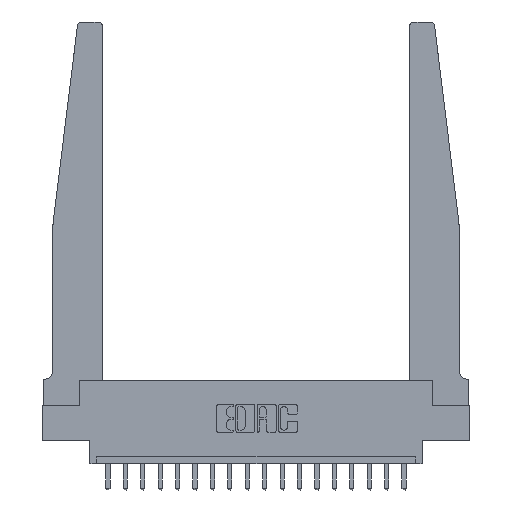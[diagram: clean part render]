
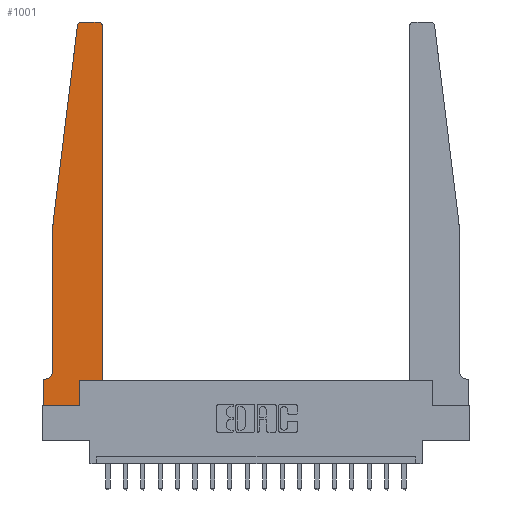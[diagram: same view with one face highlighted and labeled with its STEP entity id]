
A CAD part, top view. The second image highlights one B-rep face of the part: STEP entity #1001.
In plain terms, the highlighted planar face has unit normal (0, 0, 1).
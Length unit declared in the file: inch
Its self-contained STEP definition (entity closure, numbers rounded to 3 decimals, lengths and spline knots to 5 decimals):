
#189 = CARTESIAN_POINT ( 'NONE',  ( 0.425, 2.72, 0.37 ) ) ;
#307 = VERTEX_POINT ( 'NONE', #17129 ) ;
#1001 = ADVANCED_FACE ( 'NONE', ( #6312 ), #4808, .T. ) ;
#1049 = LINE ( 'NONE', #13398, #4897 ) ;
#1260 = EDGE_CURVE ( 'NONE', #4335, #16055, #1049, .T. ) ;
#1271 = ORIENTED_EDGE ( 'NONE', *, *, #1260, .T. ) ;
#1694 = ORIENTED_EDGE ( 'NONE', *, *, #8791, .T. ) ;
#1933 = LINE ( 'NONE', #2141, #8858 ) ;
#2081 = EDGE_CURVE ( 'NONE', #16055, #9278, #18483, .T. ) ;
#2141 = CARTESIAN_POINT ( 'NONE',  ( 0.065, 1.25, 0.37 ) ) ;
#2741 = CARTESIAN_POINT ( 'NONE',  ( 0.24675, 2.72367, 0.37 ) ) ;
#2771 = DIRECTION ( 'NONE',  ( 0., 1., 0. ) ) ;
#2878 = DIRECTION ( 'NONE',  ( 1., 0., 0. ) ) ;
#2990 = CARTESIAN_POINT ( 'NONE',  ( 0., 0., 0.37 ) ) ;
#3094 = DIRECTION ( 'NONE',  ( 0., -1., 0. ) ) ;
#3501 = DIRECTION ( 'NONE',  ( -1., 0., 0. ) ) ;
#3681 = AXIS2_PLACEMENT_3D ( 'NONE', #15258, #10848, #9333 ) ;
#3747 = CARTESIAN_POINT ( 'NONE',  ( 0.015, 0.1875, 0.37 ) ) ;
#3793 = LINE ( 'NONE', #9894, #6605 ) ;
#3948 = VERTEX_POINT ( 'NONE', #5786 ) ;
#4172 = CARTESIAN_POINT ( 'NONE',  ( 0.065, 0.2375, 0.37 ) ) ;
#4216 = VECTOR ( 'NONE', #16671, 39.37008 ) ;
#4335 = VERTEX_POINT ( 'NONE', #8942 ) ;
#4771 = CARTESIAN_POINT ( 'NONE',  ( 0.065, 1.25, 0.37 ) ) ;
#4808 = PLANE ( 'NONE',  #17372 ) ;
#4897 = VECTOR ( 'NONE', #2878, 39.37008 ) ;
#5011 = LINE ( 'NONE', #19052, #19082 ) ;
#5083 = DIRECTION ( 'NONE',  ( 1., 0., 0. ) ) ;
#5173 = DIRECTION ( 'NONE',  ( 0., -1., 0. ) ) ;
#5688 = DIRECTION ( 'NONE',  ( 0., 0., 1. ) ) ;
#5760 = VECTOR ( 'NONE', #3094, 39.37008 ) ;
#5786 = CARTESIAN_POINT ( 'NONE',  ( 0.2605, 0., 0.37 ) ) ;
#5895 = CIRCLE ( 'NONE', #3681, 0.05 ) ;
#5981 = CARTESIAN_POINT ( 'NONE',  ( 0.2605, 0.18, 0.37 ) ) ;
#6050 = CARTESIAN_POINT ( 'NONE',  ( 0.425, 0.18, 0.37 ) ) ;
#6312 = FACE_OUTER_BOUND ( 'NONE', #16647, .T. ) ;
#6335 = CARTESIAN_POINT ( 'NONE',  ( 0.425, 0.18, 0.37 ) ) ;
#6598 = ORIENTED_EDGE ( 'NONE', *, *, #17823, .T. ) ;
#6605 = VECTOR ( 'NONE', #16205, 39.37008 ) ;
#7017 = EDGE_CURVE ( 'NONE', #15903, #14221, #15276, .T. ) ;
#7589 = LINE ( 'NONE', #2990, #5760 ) ;
#8445 = EDGE_CURVE ( 'NONE', #14431, #10564, #7589, .T. ) ;
#8791 = EDGE_CURVE ( 'NONE', #10753, #14431, #3793, .T. ) ;
#8858 = VECTOR ( 'NONE', #5173, 39.37008 ) ;
#8942 = CARTESIAN_POINT ( 'NONE',  ( 0.2605, 0.18, 0.37 ) ) ;
#9002 = DIRECTION ( 'NONE',  ( 0., 0., 1. ) ) ;
#9048 = DIRECTION ( 'NONE',  ( -0.122, -0.992, 0. ) ) ;
#9147 = CARTESIAN_POINT ( 'NONE',  ( 0., 0., 0.37 ) ) ;
#9205 = VECTOR ( 'NONE', #9048, 39.37008 ) ;
#9232 = DIRECTION ( 'NONE',  ( 0., 1., 0. ) ) ;
#9278 = VERTEX_POINT ( 'NONE', #189 ) ;
#9333 = DIRECTION ( 'NONE',  ( -1., 0., 0. ) ) ;
#9409 = DIRECTION ( 'NONE',  ( 1., 0., 0. ) ) ;
#9869 = CARTESIAN_POINT ( 'NONE',  ( 0.27653, 2.72, 0.37 ) ) ;
#9894 = CARTESIAN_POINT ( 'NONE',  ( 0.065, 0.1875, 0.37 ) ) ;
#10564 = VERTEX_POINT ( 'NONE', #9147 ) ;
#10649 = CARTESIAN_POINT ( 'NONE',  ( 0., 0., 0.37 ) ) ;
#10753 = VERTEX_POINT ( 'NONE', #3747 ) ;
#10848 = DIRECTION ( 'NONE',  ( 0., 0., -1. ) ) ;
#11029 = AXIS2_PLACEMENT_3D ( 'NONE', #11491, #5688, #17940 ) ;
#11058 = EDGE_CURVE ( 'NONE', #307, #13666, #5011, .T. ) ;
#11218 = CARTESIAN_POINT ( 'NONE',  ( 0.27653, 2.75, 0.37 ) ) ;
#11281 = EDGE_CURVE ( 'NONE', #9278, #307, #14230, .T. ) ;
#11335 = EDGE_CURVE ( 'NONE', #3948, #4335, #16503, .T. ) ;
#11491 = CARTESIAN_POINT ( 'NONE',  ( 0.395, 2.72, 0.37 ) ) ;
#12615 = VECTOR ( 'NONE', #2771, 39.37008 ) ;
#12963 = EDGE_CURVE ( 'NONE', #17239, #10753, #5895, .T. ) ;
#13045 = ORIENTED_EDGE ( 'NONE', *, *, #14447, .T. ) ;
#13398 = CARTESIAN_POINT ( 'NONE',  ( 0.425, 0.18, 0.37 ) ) ;
#13666 = VERTEX_POINT ( 'NONE', #11218 ) ;
#13668 = ORIENTED_EDGE ( 'NONE', *, *, #11335, .T. ) ;
#13903 = VECTOR ( 'NONE', #9232, 39.37008 ) ;
#14221 = VERTEX_POINT ( 'NONE', #4771 ) ;
#14230 = CIRCLE ( 'NONE', #11029, 0.03 ) ;
#14431 = VERTEX_POINT ( 'NONE', #18919 ) ;
#14447 = EDGE_CURVE ( 'NONE', #14221, #17239, #1933, .T. ) ;
#14472 = ORIENTED_EDGE ( 'NONE', *, *, #7017, .T. ) ;
#15258 = CARTESIAN_POINT ( 'NONE',  ( 0.015, 0.2375, 0.37 ) ) ;
#15276 = LINE ( 'NONE', #15485, #9205 ) ;
#15485 = CARTESIAN_POINT ( 'NONE',  ( 0.065, 1.25, 0.37 ) ) ;
#15810 = CARTESIAN_POINT ( 'NONE',  ( 0., 0.1875, 0.37 ) ) ;
#15883 = ORIENTED_EDGE ( 'NONE', *, *, #8445, .T. ) ;
#15903 = VERTEX_POINT ( 'NONE', #2741 ) ;
#16051 = CIRCLE ( 'NONE', #17041, 0.03 ) ;
#16055 = VERTEX_POINT ( 'NONE', #6050 ) ;
#16205 = DIRECTION ( 'NONE',  ( -1., 0., 0. ) ) ;
#16503 = LINE ( 'NONE', #5981, #12615 ) ;
#16537 = ORIENTED_EDGE ( 'NONE', *, *, #11281, .T. ) ;
#16647 = EDGE_LOOP ( 'NONE', ( #18534, #18192, #14472, #13045, #17179, #1694, #15883, #6598, #13668, #1271, #19428, #16537 ) ) ;
#16671 = DIRECTION ( 'NONE',  ( 1., 0., 0. ) ) ;
#17041 = AXIS2_PLACEMENT_3D ( 'NONE', #9869, #18822, #5083 ) ;
#17129 = CARTESIAN_POINT ( 'NONE',  ( 0.395, 2.75, 0.37 ) ) ;
#17179 = ORIENTED_EDGE ( 'NONE', *, *, #12963, .T. ) ;
#17239 = VERTEX_POINT ( 'NONE', #4172 ) ;
#17372 = AXIS2_PLACEMENT_3D ( 'NONE', #15810, #9002, #9409 ) ;
#17532 = EDGE_CURVE ( 'NONE', #13666, #15903, #16051, .T. ) ;
#17823 = EDGE_CURVE ( 'NONE', #10564, #3948, #19708, .T. ) ;
#17940 = DIRECTION ( 'NONE',  ( 1., 0., 0. ) ) ;
#18192 = ORIENTED_EDGE ( 'NONE', *, *, #17532, .T. ) ;
#18483 = LINE ( 'NONE', #6335, #13903 ) ;
#18534 = ORIENTED_EDGE ( 'NONE', *, *, #11058, .T. ) ;
#18822 = DIRECTION ( 'NONE',  ( 0., 0., 1. ) ) ;
#18919 = CARTESIAN_POINT ( 'NONE',  ( 0., 0.1875, 0.37 ) ) ;
#19052 = CARTESIAN_POINT ( 'NONE',  ( 0.25, 2.75, 0.37 ) ) ;
#19082 = VECTOR ( 'NONE', #3501, 39.37008 ) ;
#19428 = ORIENTED_EDGE ( 'NONE', *, *, #2081, .T. ) ;
#19708 = LINE ( 'NONE', #10649, #4216 ) ;
